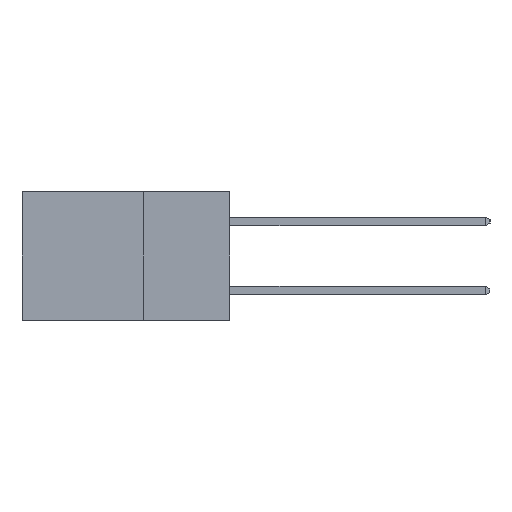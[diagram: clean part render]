
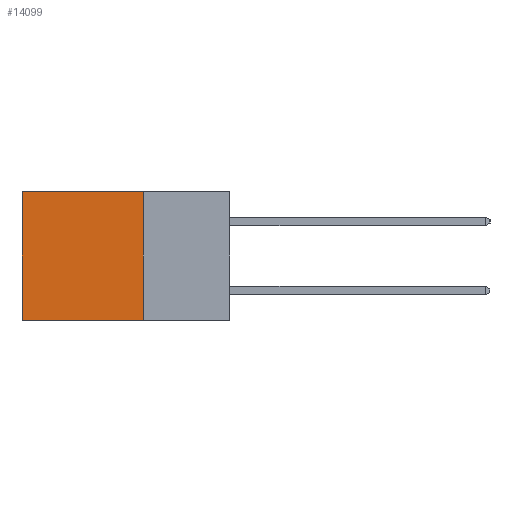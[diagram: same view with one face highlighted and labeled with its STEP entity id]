
A CAD part, left-side view. The second image highlights one B-rep face of the part: STEP entity #14099.
In plain terms, the highlighted planar face has unit normal (-1, 0, 0).
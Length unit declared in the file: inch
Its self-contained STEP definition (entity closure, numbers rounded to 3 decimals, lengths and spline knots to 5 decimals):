
#148 = ORIENTED_EDGE ( 'NONE', *, *, #873, .F. ) ;
#291 = ORIENTED_EDGE ( 'NONE', *, *, #15010, .T. ) ;
#487 = CARTESIAN_POINT ( 'NONE',  ( 0.298, 0.6, 0. ) ) ;
#563 = CARTESIAN_POINT ( 'NONE',  ( 0.298, 0.25, 0. ) ) ;
#567 = AXIS2_PLACEMENT_3D ( 'NONE', #563, #7131, #16255 ) ;
#636 = CARTESIAN_POINT ( 'NONE',  ( 0.298, 0.6, -0.37 ) ) ;
#836 = LINE ( 'NONE', #7401, #10837 ) ;
#873 = EDGE_CURVE ( 'NONE', #10972, #3619, #8862, .T. ) ;
#1917 = VECTOR ( 'NONE', #13368, 39.37008 ) ;
#2274 = CARTESIAN_POINT ( 'NONE',  ( 0.298, 0.25, 0. ) ) ;
#2395 = CARTESIAN_POINT ( 'NONE',  ( 0.298, 0.25, -0.37 ) ) ;
#3619 = VERTEX_POINT ( 'NONE', #2395 ) ;
#6062 = VERTEX_POINT ( 'NONE', #636 ) ;
#6445 = VECTOR ( 'NONE', #8283, 39.37008 ) ;
#7131 = DIRECTION ( 'NONE',  ( 1., 0., 0. ) ) ;
#7231 = EDGE_CURVE ( 'NONE', #3619, #6062, #836, .T. ) ;
#7401 = CARTESIAN_POINT ( 'NONE',  ( 0.298, 0.25, -0.37 ) ) ;
#7499 = DIRECTION ( 'NONE',  ( 0., 1., 0. ) ) ;
#7718 = CARTESIAN_POINT ( 'NONE',  ( 0.298, 0.25, 0. ) ) ;
#8280 = LINE ( 'NONE', #7718, #14412 ) ;
#8283 = DIRECTION ( 'NONE',  ( 0., 0., -1. ) ) ;
#8862 = LINE ( 'NONE', #12321, #1917 ) ;
#9084 = DIRECTION ( 'NONE',  ( 0., 1., 0. ) ) ;
#10286 = FACE_OUTER_BOUND ( 'NONE', #13441, .T. ) ;
#10410 = VERTEX_POINT ( 'NONE', #11436 ) ;
#10837 = VECTOR ( 'NONE', #7499, 39.37008 ) ;
#10972 = VERTEX_POINT ( 'NONE', #2274 ) ;
#11436 = CARTESIAN_POINT ( 'NONE',  ( 0.298, 0.6, 0. ) ) ;
#12321 = CARTESIAN_POINT ( 'NONE',  ( 0.298, 0.25, 0. ) ) ;
#13368 = DIRECTION ( 'NONE',  ( 0., 0., -1. ) ) ;
#13441 = EDGE_LOOP ( 'NONE', ( #15295, #14879, #148, #291 ) ) ;
#14099 = ADVANCED_FACE ( 'NONE', ( #10286 ), #14916, .F. ) ;
#14412 = VECTOR ( 'NONE', #9084, 39.37008 ) ;
#14879 = ORIENTED_EDGE ( 'NONE', *, *, #7231, .F. ) ;
#14916 = PLANE ( 'NONE',  #567 ) ;
#15010 = EDGE_CURVE ( 'NONE', #10972, #10410, #8280, .T. ) ;
#15295 = ORIENTED_EDGE ( 'NONE', *, *, #15296, .T. ) ;
#15296 = EDGE_CURVE ( 'NONE', #10410, #6062, #16840, .T. ) ;
#16255 = DIRECTION ( 'NONE',  ( 0., 0., -1. ) ) ;
#16840 = LINE ( 'NONE', #487, #6445 ) ;
